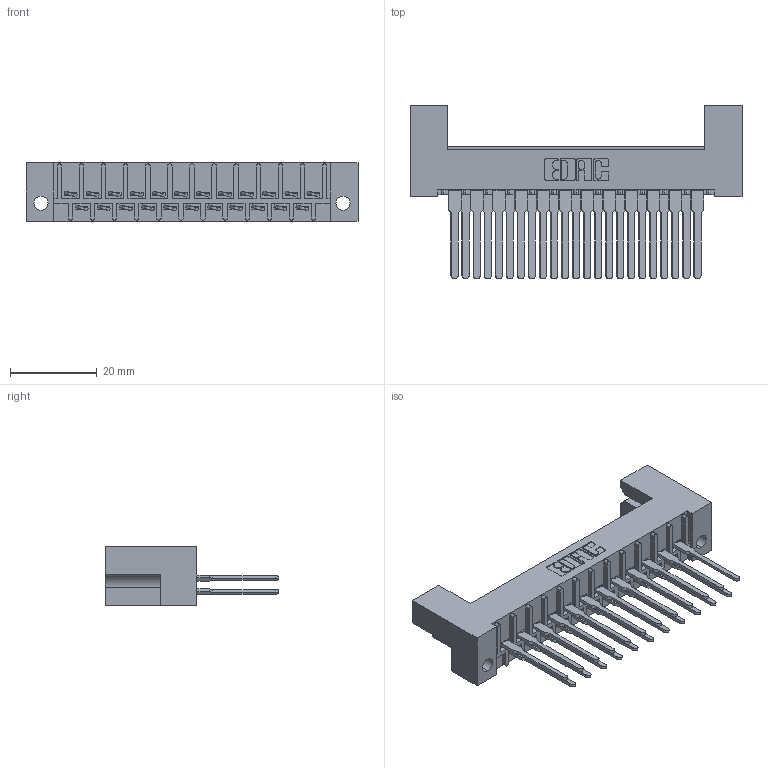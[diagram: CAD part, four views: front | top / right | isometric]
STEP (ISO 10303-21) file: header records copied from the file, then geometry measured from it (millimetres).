
FILE_DESCRIPTION (( 'STEP AP203' ), '1' );
FILE_NAME ('408-023-541-222.STEP', '2019-11-04T18:51:57', ( '' ), ( '' ), 'SwSTEP 2.0', 'SolidWorks 2016', '' );
FILE_SCHEMA (( 'CONFIG_CONTROL_DESIGN' ));
Length unit declared in the file: inch
Products named in the file (3): 408-023-541-222; 408-290-001_408-290-141; 408 Part_023 - 2
Assembly tree (24 placements, depth 2):
  408-023-541-222
    408 Part_023 - 2
    408-290-001_408-290-141  x23
Bounding box: 76.35 x 39.93 x 13.49 mm (x, y, z)
Volume: 10361.1 mm3; surface area: 12684.3 mm2
Topology: 24 solids, 24 shells, 1358 faces, 3724 edges, 2420 vertices
Faces by surface type: plane 1009, cylinder 257, bspline 92
Entity records: 19693 total; most frequent: CARTESIAN_POINT 3405, ORIENTED_EDGE 3312, DIRECTION 3032, EDGE_CURVE 1656, LINE 1450, VECTOR 1450, VERTEX_POINT 1100, AXIS2_PLACEMENT_3D 791
